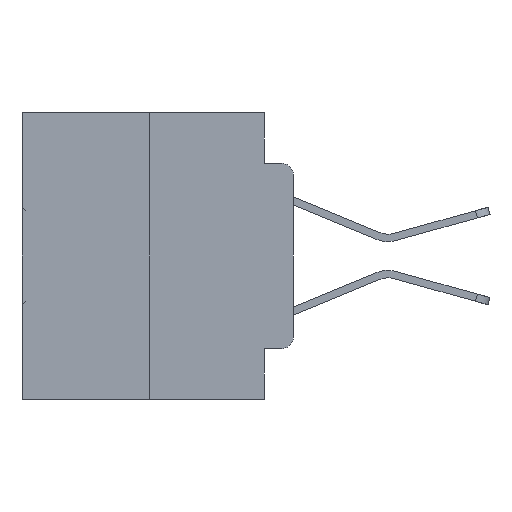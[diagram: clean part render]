
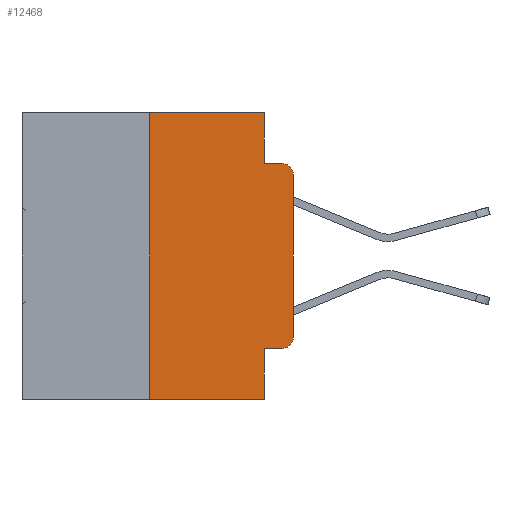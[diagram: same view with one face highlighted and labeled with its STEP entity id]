
A CAD part, left-side view. The second image highlights one B-rep face of the part: STEP entity #12468.
In plain terms, the highlighted planar face has unit normal (-1, 0, 0).
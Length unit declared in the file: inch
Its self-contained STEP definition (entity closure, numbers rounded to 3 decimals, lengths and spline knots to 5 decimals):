
#40 = FACE_OUTER_BOUND ( 'NONE', #954, .T. ) ;
#241 = CARTESIAN_POINT ( 'NONE',  ( 0., 0., 0. ) ) ;
#439 = ORIENTED_EDGE ( 'NONE', *, *, #12627, .F. ) ;
#629 = CARTESIAN_POINT ( 'NONE',  ( 0., 0.051, -0.4115 ) ) ;
#704 = AXIS2_PLACEMENT_3D ( 'NONE', #24226, #9220, #26719 ) ;
#954 = EDGE_LOOP ( 'NONE', ( #3176, #1930, #439, #1002, #1632, #4046, #4335, #6812, #16967, #9041 ) ) ;
#1002 = ORIENTED_EDGE ( 'NONE', *, *, #9124, .F. ) ;
#1008 = CARTESIAN_POINT ( 'NONE',  ( 0., 0.473, -0.5 ) ) ;
#1058 = VECTOR ( 'NONE', #8334, 39.37008 ) ;
#1632 = ORIENTED_EDGE ( 'NONE', *, *, #31858, .F. ) ;
#1930 = ORIENTED_EDGE ( 'NONE', *, *, #12586, .T. ) ;
#3071 = VERTEX_POINT ( 'NONE', #5861 ) ;
#3176 = ORIENTED_EDGE ( 'NONE', *, *, #18139, .T. ) ;
#3668 = VECTOR ( 'NONE', #25169, 39.37008 ) ;
#3700 = EDGE_CURVE ( 'NONE', #5127, #26161, #16064, .T. ) ;
#4046 = ORIENTED_EDGE ( 'NONE', *, *, #15454, .F. ) ;
#4093 = VERTEX_POINT ( 'NONE', #14288 ) ;
#4133 = VERTEX_POINT ( 'NONE', #4232 ) ;
#4147 = CARTESIAN_POINT ( 'NONE',  ( 0., 0.02, -0.0885 ) ) ;
#4232 = CARTESIAN_POINT ( 'NONE',  ( 0., 0.25, 0. ) ) ;
#4335 = ORIENTED_EDGE ( 'NONE', *, *, #26850, .T. ) ;
#5069 = DIRECTION ( 'NONE',  ( -1., 0., 0. ) ) ;
#5127 = VERTEX_POINT ( 'NONE', #629 ) ;
#5861 = CARTESIAN_POINT ( 'NONE',  ( 0., 0., -0.1085 ) ) ;
#6812 = ORIENTED_EDGE ( 'NONE', *, *, #15433, .F. ) ;
#7721 = CARTESIAN_POINT ( 'NONE',  ( 0., 0.051, -0.0885 ) ) ;
#7848 = LINE ( 'NONE', #20890, #1058 ) ;
#7866 = CARTESIAN_POINT ( 'NONE',  ( 0., 0.02, -0.4115 ) ) ;
#8334 = DIRECTION ( 'NONE',  ( 0., 0., -1. ) ) ;
#8542 = VECTOR ( 'NONE', #22451, 39.37008 ) ;
#9041 = ORIENTED_EDGE ( 'NONE', *, *, #28237, .T. ) ;
#9124 = EDGE_CURVE ( 'NONE', #29684, #30562, #26210, .T. ) ;
#9220 = DIRECTION ( 'NONE',  ( -1., 0., 0. ) ) ;
#9395 = CARTESIAN_POINT ( 'NONE',  ( 0., 0.051, -0.5 ) ) ;
#11456 = LINE ( 'NONE', #22763, #23954 ) ;
#11864 = VERTEX_POINT ( 'NONE', #4147 ) ;
#11961 = CIRCLE ( 'NONE', #27312, 0.02 ) ;
#12096 = DIRECTION ( 'NONE',  ( 1., 0., 0. ) ) ;
#12221 = VERTEX_POINT ( 'NONE', #18840 ) ;
#12468 = ADVANCED_FACE ( 'NONE', ( #40 ), #22072, .F. ) ;
#12586 = EDGE_CURVE ( 'NONE', #3071, #11864, #11961, .T. ) ;
#12627 = EDGE_CURVE ( 'NONE', #30562, #11864, #16307, .T. ) ;
#14288 = CARTESIAN_POINT ( 'NONE',  ( 0., 0., -0.3915 ) ) ;
#14492 = CIRCLE ( 'NONE', #704, 0.02 ) ;
#14552 = LINE ( 'NONE', #25822, #20427 ) ;
#14590 = VECTOR ( 'NONE', #21192, 39.37008 ) ;
#15433 = EDGE_CURVE ( 'NONE', #5127, #15693, #7848, .T. ) ;
#15454 = EDGE_CURVE ( 'NONE', #12221, #4133, #14552, .T. ) ;
#15680 = AXIS2_PLACEMENT_3D ( 'NONE', #27017, #12096, #29523 ) ;
#15693 = VERTEX_POINT ( 'NONE', #9395 ) ;
#16064 = LINE ( 'NONE', #27741, #8542 ) ;
#16307 = LINE ( 'NONE', #7721, #3668 ) ;
#16967 = ORIENTED_EDGE ( 'NONE', *, *, #3700, .T. ) ;
#17193 = VECTOR ( 'NONE', #17968, 39.37008 ) ;
#17968 = DIRECTION ( 'NONE',  ( 0., 0., 1. ) ) ;
#18139 = EDGE_CURVE ( 'NONE', #4093, #3071, #29583, .T. ) ;
#18840 = CARTESIAN_POINT ( 'NONE',  ( 0., 0.25, -0.5 ) ) ;
#19665 = VECTOR ( 'NONE', #26667, 39.37008 ) ;
#20140 = CARTESIAN_POINT ( 'NONE',  ( 0., 0.02, -0.1085 ) ) ;
#20427 = VECTOR ( 'NONE', #30814, 39.37008 ) ;
#20890 = CARTESIAN_POINT ( 'NONE',  ( 0., 0.051, 0. ) ) ;
#21192 = DIRECTION ( 'NONE',  ( 0., -1., 0. ) ) ;
#21229 = LINE ( 'NONE', #1008, #14590 ) ;
#21286 = CARTESIAN_POINT ( 'NONE',  ( 0., 0.051, 0. ) ) ;
#22072 = PLANE ( 'NONE',  #15680 ) ;
#22451 = DIRECTION ( 'NONE',  ( 0., -1., 0. ) ) ;
#22588 = DIRECTION ( 'NONE',  ( 0., 0., -1. ) ) ;
#22763 = CARTESIAN_POINT ( 'NONE',  ( 0., 0.473, 0. ) ) ;
#23954 = VECTOR ( 'NONE', #25238, 39.37008 ) ;
#24226 = CARTESIAN_POINT ( 'NONE',  ( 0., 0.02, -0.3915 ) ) ;
#25169 = DIRECTION ( 'NONE',  ( 0., -1., 0. ) ) ;
#25238 = DIRECTION ( 'NONE',  ( 0., -1., 0. ) ) ;
#25822 = CARTESIAN_POINT ( 'NONE',  ( 0., 0.25, 0. ) ) ;
#26161 = VERTEX_POINT ( 'NONE', #7866 ) ;
#26210 = LINE ( 'NONE', #26236, #19665 ) ;
#26236 = CARTESIAN_POINT ( 'NONE',  ( 0., 0.051, 0. ) ) ;
#26667 = DIRECTION ( 'NONE',  ( 0., 0., -1. ) ) ;
#26719 = DIRECTION ( 'NONE',  ( 0., 0., -1. ) ) ;
#26850 = EDGE_CURVE ( 'NONE', #12221, #15693, #21229, .T. ) ;
#27017 = CARTESIAN_POINT ( 'NONE',  ( 0., 0.473, 0. ) ) ;
#27312 = AXIS2_PLACEMENT_3D ( 'NONE', #20140, #5069, #22588 ) ;
#27741 = CARTESIAN_POINT ( 'NONE',  ( 0., 0.051, -0.4115 ) ) ;
#28237 = EDGE_CURVE ( 'NONE', #26161, #4093, #14492, .T. ) ;
#29523 = DIRECTION ( 'NONE',  ( 0., 0., -1. ) ) ;
#29583 = LINE ( 'NONE', #241, #17193 ) ;
#29684 = VERTEX_POINT ( 'NONE', #21286 ) ;
#29988 = CARTESIAN_POINT ( 'NONE',  ( 0., 0.051, -0.0885 ) ) ;
#30562 = VERTEX_POINT ( 'NONE', #29988 ) ;
#30814 = DIRECTION ( 'NONE',  ( 0., 0., 1. ) ) ;
#31858 = EDGE_CURVE ( 'NONE', #4133, #29684, #11456, .T. ) ;
